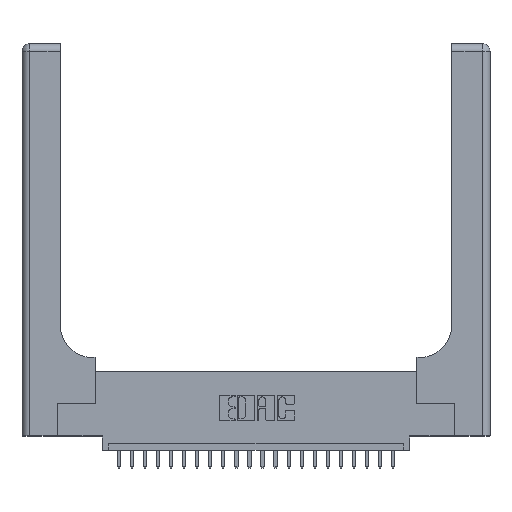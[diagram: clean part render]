
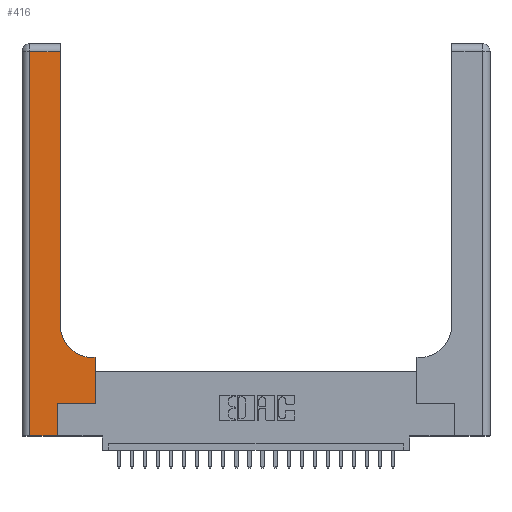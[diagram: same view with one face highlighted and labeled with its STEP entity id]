
A CAD part, top view. The second image highlights one B-rep face of the part: STEP entity #416.
In plain terms, the highlighted planar face has unit normal (0, 0, 1).
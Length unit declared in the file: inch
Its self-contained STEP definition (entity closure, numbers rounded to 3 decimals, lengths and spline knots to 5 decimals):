
#34 = DIRECTION ( 'NONE',  ( 0., 0., -1. ) ) ;
#353 = EDGE_CURVE ( 'NONE', #1127, #9681, #4149, .T. ) ;
#416 = ADVANCED_FACE ( 'NONE', ( #9160 ), #14697, .F. ) ;
#521 = ORIENTED_EDGE ( 'NONE', *, *, #3839, .T. ) ;
#673 = DIRECTION ( 'NONE',  ( 0., -1., 0. ) ) ;
#1065 = VERTEX_POINT ( 'NONE', #10997 ) ;
#1079 = ORIENTED_EDGE ( 'NONE', *, *, #20567, .T. ) ;
#1127 = VERTEX_POINT ( 'NONE', #24362 ) ;
#1223 = DIRECTION ( 'NONE',  ( 1., 0., 0. ) ) ;
#1281 = ORIENTED_EDGE ( 'NONE', *, *, #11260, .T. ) ;
#1330 = EDGE_CURVE ( 'NONE', #12623, #1127, #11823, .T. ) ;
#1370 = CARTESIAN_POINT ( 'NONE',  ( 0.5585, 0.25, 0.37 ) ) ;
#1838 = ORIENTED_EDGE ( 'NONE', *, *, #19826, .T. ) ;
#2053 = ORIENTED_EDGE ( 'NONE', *, *, #1330, .T. ) ;
#2156 = DIRECTION ( 'NONE',  ( -1., 0., 0. ) ) ;
#2364 = LINE ( 'NONE', #3457, #14218 ) ;
#2696 = EDGE_LOOP ( 'NONE', ( #2053, #13463, #1079, #521, #7044, #18503, #1281, #7950, #1838 ) ) ;
#2931 = CARTESIAN_POINT ( 'NONE',  ( 0.06, 2.94, 0.37 ) ) ;
#3039 = AXIS2_PLACEMENT_3D ( 'NONE', #4132, #34, #19059 ) ;
#3457 = CARTESIAN_POINT ( 'NONE',  ( 0.269, 0.25, 0.37 ) ) ;
#3583 = DIRECTION ( 'NONE',  ( 0., 1., 0. ) ) ;
#3839 = EDGE_CURVE ( 'NONE', #7094, #1065, #9032, .T. ) ;
#4132 = CARTESIAN_POINT ( 'NONE',  ( 0.5415, 0.85, 0.37 ) ) ;
#4149 = LINE ( 'NONE', #16096, #15085 ) ;
#4579 = VECTOR ( 'NONE', #2156, 39.37008 ) ;
#7044 = ORIENTED_EDGE ( 'NONE', *, *, #9609, .T. ) ;
#7094 = VERTEX_POINT ( 'NONE', #16780 ) ;
#7263 = CARTESIAN_POINT ( 'NONE',  ( 0.5585, 0.25, 0.37 ) ) ;
#7758 = VECTOR ( 'NONE', #3583, 39.37008 ) ;
#7950 = ORIENTED_EDGE ( 'NONE', *, *, #10196, .T. ) ;
#8310 = DIRECTION ( 'NONE',  ( 0., 1., 0. ) ) ;
#8695 = DIRECTION ( 'NONE',  ( 0., 0., -1. ) ) ;
#9032 = LINE ( 'NONE', #22046, #23027 ) ;
#9160 = FACE_OUTER_BOUND ( 'NONE', #2696, .T. ) ;
#9609 = EDGE_CURVE ( 'NONE', #1065, #20138, #9885, .T. ) ;
#9681 = VERTEX_POINT ( 'NONE', #2931 ) ;
#9885 = LINE ( 'NONE', #23583, #18495 ) ;
#10196 = EDGE_CURVE ( 'NONE', #16260, #10333, #21777, .T. ) ;
#10333 = VERTEX_POINT ( 'NONE', #18057 ) ;
#10997 = CARTESIAN_POINT ( 'NONE',  ( 0.269, 0., 0.37 ) ) ;
#11260 = EDGE_CURVE ( 'NONE', #14905, #16260, #15168, .T. ) ;
#11823 = LINE ( 'NONE', #17527, #20768 ) ;
#12623 = VERTEX_POINT ( 'NONE', #14512 ) ;
#13322 = CIRCLE ( 'NONE', #3039, 0.25 ) ;
#13463 = ORIENTED_EDGE ( 'NONE', *, *, #353, .T. ) ;
#14218 = VECTOR ( 'NONE', #14895, 39.37008 ) ;
#14512 = CARTESIAN_POINT ( 'NONE',  ( 0.2915, 0.85, 0.37 ) ) ;
#14697 = PLANE ( 'NONE',  #19972 ) ;
#14895 = DIRECTION ( 'NONE',  ( 1., 0., 0. ) ) ;
#14905 = VERTEX_POINT ( 'NONE', #1370 ) ;
#15085 = VECTOR ( 'NONE', #23731, 39.37008 ) ;
#15168 = LINE ( 'NONE', #7263, #7758 ) ;
#15299 = CARTESIAN_POINT ( 'NONE',  ( 0.2915, 0.6, 0.37 ) ) ;
#16096 = CARTESIAN_POINT ( 'NONE',  ( 0., 2.94, 0.37 ) ) ;
#16260 = VERTEX_POINT ( 'NONE', #23929 ) ;
#16294 = EDGE_CURVE ( 'NONE', #20138, #14905, #2364, .T. ) ;
#16512 = CARTESIAN_POINT ( 'NONE',  ( 0.269, 0.25, 0.37 ) ) ;
#16665 = CARTESIAN_POINT ( 'NONE',  ( 0., 3., 0.37 ) ) ;
#16780 = CARTESIAN_POINT ( 'NONE',  ( 0.06, 0., 0.37 ) ) ;
#17527 = CARTESIAN_POINT ( 'NONE',  ( 0.2915, 3., 0.37 ) ) ;
#18057 = CARTESIAN_POINT ( 'NONE',  ( 0.5415, 0.6, 0.37 ) ) ;
#18495 = VECTOR ( 'NONE', #8310, 39.37008 ) ;
#18503 = ORIENTED_EDGE ( 'NONE', *, *, #16294, .T. ) ;
#19059 = DIRECTION ( 'NONE',  ( 1., 0., 0. ) ) ;
#19826 = EDGE_CURVE ( 'NONE', #10333, #12623, #13322, .T. ) ;
#19972 = AXIS2_PLACEMENT_3D ( 'NONE', #16665, #8695, #20248 ) ;
#20138 = VERTEX_POINT ( 'NONE', #16512 ) ;
#20248 = DIRECTION ( 'NONE',  ( -1., 0., 0. ) ) ;
#20567 = EDGE_CURVE ( 'NONE', #9681, #7094, #21242, .T. ) ;
#20768 = VECTOR ( 'NONE', #23344, 39.37008 ) ;
#21242 = LINE ( 'NONE', #21424, #21833 ) ;
#21424 = CARTESIAN_POINT ( 'NONE',  ( 0.06, 3., 0.37 ) ) ;
#21777 = LINE ( 'NONE', #15299, #4579 ) ;
#21833 = VECTOR ( 'NONE', #673, 39.37008 ) ;
#22046 = CARTESIAN_POINT ( 'NONE',  ( 0., 0., 0.37 ) ) ;
#23027 = VECTOR ( 'NONE', #1223, 39.37008 ) ;
#23344 = DIRECTION ( 'NONE',  ( 0., 1., 0. ) ) ;
#23583 = CARTESIAN_POINT ( 'NONE',  ( 0.269, 0., 0.37 ) ) ;
#23731 = DIRECTION ( 'NONE',  ( -1., 0., 0. ) ) ;
#23929 = CARTESIAN_POINT ( 'NONE',  ( 0.5585, 0.6, 0.37 ) ) ;
#24362 = CARTESIAN_POINT ( 'NONE',  ( 0.2915, 2.94, 0.37 ) ) ;
